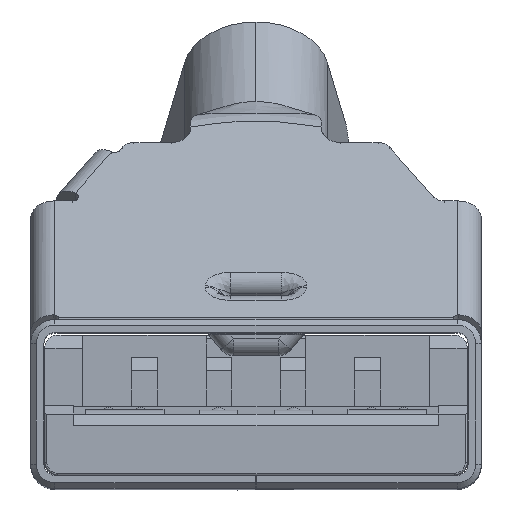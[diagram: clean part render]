
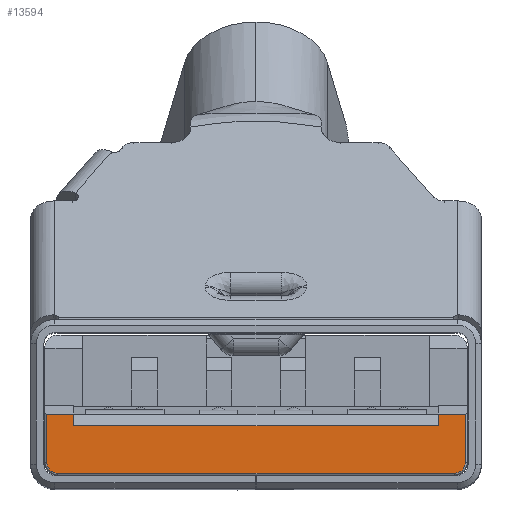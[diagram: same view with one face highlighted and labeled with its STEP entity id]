
A CAD part, top view. The second image highlights one B-rep face of the part: STEP entity #13594.
In plain terms, the highlighted face is planar.
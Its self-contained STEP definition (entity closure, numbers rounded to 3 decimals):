
#228 = ORIENTED_EDGE ( 'NONE', *, *, #15089, .T. ) ;
#372 = ORIENTED_EDGE ( 'NONE', *, *, #15544, .T. ) ;
#379 = CARTESIAN_POINT ( 'NONE',  ( -5.575, 8.5, 0.27 ) ) ;
#1093 = CARTESIAN_POINT ( 'NONE',  ( -5.575, 8.5, 0.84 ) ) ;
#1177 = CARTESIAN_POINT ( 'NONE',  ( -4.85, 8.5, 1.63 ) ) ;
#1186 = CARTESIAN_POINT ( 'NONE',  ( 5.575, 8.5, 1.63 ) ) ;
#2234 = CARTESIAN_POINT ( 'NONE',  ( 4.85, 8.5, 1.63 ) ) ;
#3804 = ORIENTED_EDGE ( 'NONE', *, *, #37440, .T. ) ;
#4508 = VERTEX_POINT ( 'NONE', #7516 ) ;
#4862 = LINE ( 'NONE', #21508, #26617 ) ;
#4922 = ORIENTED_EDGE ( 'NONE', *, *, #17686, .T. ) ;
#5712 = CARTESIAN_POINT ( 'NONE',  ( 5.575, 8.5, 0.35 ) ) ;
#5769 = ORIENTED_EDGE ( 'NONE', *, *, #17949, .T. ) ;
#5966 = EDGE_LOOP ( 'NONE', ( #27202, #228, #5769, #372, #13174, #3804, #18555, #15774, #42509, #4922 ) ) ;
#6510 = CARTESIAN_POINT ( 'NONE',  ( -4.85, 8.5, 0.84 ) ) ;
#6813 = CARTESIAN_POINT ( 'NONE',  ( 5.275, 8.5, 0.05 ) ) ;
#7356 = DIRECTION ( 'NONE',  ( 1., 0., 0. ) ) ;
#7488 = VECTOR ( 'NONE', #24766, 1000. ) ;
#7516 = CARTESIAN_POINT ( 'NONE',  ( -5.575, 8.5, 0.35 ) ) ;
#7579 = CARTESIAN_POINT ( 'NONE',  ( 0., 8.5, 1.63 ) ) ;
#7872 = EDGE_CURVE ( 'NONE', #4508, #35122, #23600, .T. ) ;
#8327 = PLANE ( 'NONE',  #11546 ) ;
#8589 = LINE ( 'NONE', #7579, #25394 ) ;
#8946 = CARTESIAN_POINT ( 'NONE',  ( 5.575, 8.5, 0.84 ) ) ;
#8975 = CARTESIAN_POINT ( 'NONE',  ( 5.275, 8.5, 0.05 ) ) ;
#9621 = CARTESIAN_POINT ( 'NONE',  ( 5.542, 8.5, 0.193 ) ) ;
#9691 = VECTOR ( 'NONE', #41574, 1000. ) ;
#11003 = CARTESIAN_POINT ( 'NONE',  ( -5.354, 8.5, 0.05 ) ) ;
#11157 = DIRECTION ( 'NONE',  ( 0., 1., 0. ) ) ;
#11546 = AXIS2_PLACEMENT_3D ( 'NONE', #20862, #11157, #31018 ) ;
#12215 = CARTESIAN_POINT ( 'NONE',  ( 0., 8.5, 0.05 ) ) ;
#12306 = CARTESIAN_POINT ( 'NONE',  ( -5.575, 8.5, 1.63 ) ) ;
#13094 = CARTESIAN_POINT ( 'NONE',  ( 0., 8.5, 1.32 ) ) ;
#13174 = ORIENTED_EDGE ( 'NONE', *, *, #15627, .T. ) ;
#13582 = CARTESIAN_POINT ( 'NONE',  ( -5.575, 8.5, 0.35 ) ) ;
#13594 = ADVANCED_FACE ( 'NONE', ( #21071 ), #8327, .T. ) ;
#14410 = VECTOR ( 'NONE', #18905, 1000. ) ;
#14537 = VECTOR ( 'NONE', #29509, 1000. ) ;
#14782 = LINE ( 'NONE', #8946, #9691 ) ;
#14806 = VERTEX_POINT ( 'NONE', #1186 ) ;
#15089 = EDGE_CURVE ( 'NONE', #23044, #14806, #8589, .T. ) ;
#15414 = EDGE_CURVE ( 'NONE', #28221, #23044, #28218, .T. ) ;
#15544 = EDGE_CURVE ( 'NONE', #32958, #33090, #23522, .T. ) ;
#15627 = EDGE_CURVE ( 'NONE', #33090, #24322, #28623, .T. ) ;
#15774 = ORIENTED_EDGE ( 'NONE', *, *, #28065, .T. ) ;
#17466 = CARTESIAN_POINT ( 'NONE',  ( -5.275, 8.5, 0.05 ) ) ;
#17686 = EDGE_CURVE ( 'NONE', #29880, #28221, #35783, .T. ) ;
#17949 = EDGE_CURVE ( 'NONE', #14806, #32958, #14782, .T. ) ;
#18056 = DIRECTION ( 'NONE',  ( 1., 0., 0. ) ) ;
#18555 = ORIENTED_EDGE ( 'NONE', *, *, #7872, .T. ) ;
#18905 = DIRECTION ( 'NONE',  ( -1., 0., 0. ) ) ;
#20128 = DIRECTION ( 'NONE',  ( 0., 0., -1. ) ) ;
#20862 = CARTESIAN_POINT ( 'NONE',  ( 5.798, 8.5, 0.018 ) ) ;
#21071 = FACE_OUTER_BOUND ( 'NONE', #5966, .T. ) ;
#21508 = CARTESIAN_POINT ( 'NONE',  ( 0., 8.5, 1.63 ) ) ;
#21799 = VECTOR ( 'NONE', #20128, 1000. ) ;
#23044 = VERTEX_POINT ( 'NONE', #2234 ) ;
#23522 = B_SPLINE_CURVE_WITH_KNOTS ( 'NONE', 3,
 ( #5712, #25177, #9621, #35542, #42452, #8975 ),
 .UNSPECIFIED., .F., .F.,
 ( 4, 2, 4 ),
 ( 0., 0.5, 1. ),
 .UNSPECIFIED. ) ;
#23600 = LINE ( 'NONE', #1093, #29729 ) ;
#24322 = VERTEX_POINT ( 'NONE', #37743 ) ;
#24540 = CARTESIAN_POINT ( 'NONE',  ( 4.85, 8.5, 0.84 ) ) ;
#24766 = DIRECTION ( 'NONE',  ( 0., 0., 1. ) ) ;
#25177 = CARTESIAN_POINT ( 'NONE',  ( 5.575, 8.5, 0.271 ) ) ;
#25394 = VECTOR ( 'NONE', #7356, 1000. ) ;
#26617 = VECTOR ( 'NONE', #18056, 1000. ) ;
#27202 = ORIENTED_EDGE ( 'NONE', *, *, #15414, .T. ) ;
#28065 = EDGE_CURVE ( 'NONE', #35122, #28094, #4862, .T. ) ;
#28094 = VERTEX_POINT ( 'NONE', #1177 ) ;
#28218 = LINE ( 'NONE', #24540, #7488 ) ;
#28221 = VERTEX_POINT ( 'NONE', #36599 ) ;
#28623 = LINE ( 'NONE', #12215, #14410 ) ;
#29509 = DIRECTION ( 'NONE',  ( 1., 0., 0. ) ) ;
#29646 = EDGE_CURVE ( 'NONE', #28094, #29880, #42614, .T. ) ;
#29729 = VECTOR ( 'NONE', #40662, 1000. ) ;
#29880 = VERTEX_POINT ( 'NONE', #32827 ) ;
#30001 = CARTESIAN_POINT ( 'NONE',  ( -5.542, 8.5, 0.193 ) ) ;
#31018 = DIRECTION ( 'NONE',  ( -1., 0., 0. ) ) ;
#32827 = CARTESIAN_POINT ( 'NONE',  ( -4.85, 8.5, 1.32 ) ) ;
#32958 = VERTEX_POINT ( 'NONE', #35355 ) ;
#33090 = VERTEX_POINT ( 'NONE', #6813 ) ;
#33257 = CARTESIAN_POINT ( 'NONE',  ( -5.432, 8.5, 0.083 ) ) ;
#35122 = VERTEX_POINT ( 'NONE', #12306 ) ;
#35355 = CARTESIAN_POINT ( 'NONE',  ( 5.575, 8.5, 0.35 ) ) ;
#35542 = CARTESIAN_POINT ( 'NONE',  ( 5.432, 8.5, 0.083 ) ) ;
#35783 = LINE ( 'NONE', #13094, #14537 ) ;
#36599 = CARTESIAN_POINT ( 'NONE',  ( 4.85, 8.5, 1.32 ) ) ;
#37440 = EDGE_CURVE ( 'NONE', #24322, #4508, #38384, .T. ) ;
#37743 = CARTESIAN_POINT ( 'NONE',  ( -5.275, 8.5, 0.05 ) ) ;
#38384 = B_SPLINE_CURVE_WITH_KNOTS ( 'NONE', 3,
 ( #17466, #11003, #33257, #30001, #379, #13582 ),
 .UNSPECIFIED., .F., .F.,
 ( 4, 2, 4 ),
 ( 0., 0.5, 1. ),
 .UNSPECIFIED. ) ;
#40662 = DIRECTION ( 'NONE',  ( 0., 0., 1. ) ) ;
#41574 = DIRECTION ( 'NONE',  ( 0., 0., -1. ) ) ;
#42452 = CARTESIAN_POINT ( 'NONE',  ( 5.355, 8.5, 0.05 ) ) ;
#42509 = ORIENTED_EDGE ( 'NONE', *, *, #29646, .T. ) ;
#42614 = LINE ( 'NONE', #6510, #21799 ) ;
